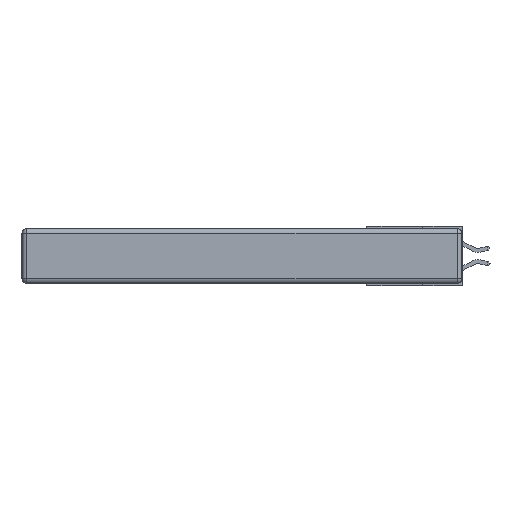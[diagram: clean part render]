
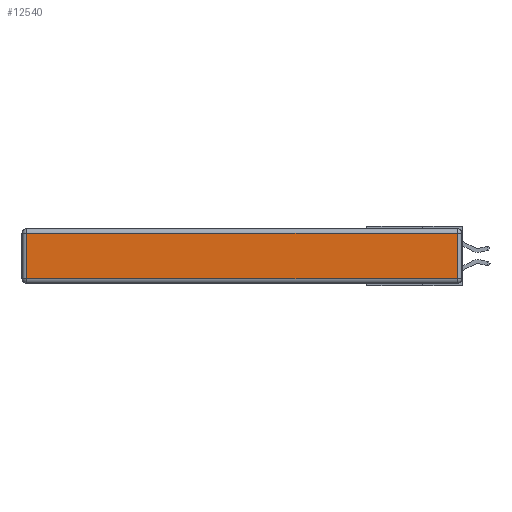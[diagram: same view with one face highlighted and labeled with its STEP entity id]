
A CAD part, left-side view. The second image highlights one B-rep face of the part: STEP entity #12540.
In plain terms, the highlighted planar face has unit normal (-1, 0, 0).
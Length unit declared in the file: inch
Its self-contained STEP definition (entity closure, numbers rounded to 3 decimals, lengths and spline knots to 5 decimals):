
#269 = VERTEX_POINT ( 'NONE', #1005 ) ;
#423 = LINE ( 'NONE', #10934, #9211 ) ;
#887 = LINE ( 'NONE', #6575, #20888 ) ;
#1005 = CARTESIAN_POINT ( 'NONE',  ( 0., 2.72, -0.313 ) ) ;
#1381 = PLANE ( 'NONE',  #4305 ) ;
#2069 = VERTEX_POINT ( 'NONE', #9112 ) ;
#3208 = DIRECTION ( 'NONE',  ( 0., 1., 0. ) ) ;
#3489 = LINE ( 'NONE', #20905, #6738 ) ;
#3576 = EDGE_CURVE ( 'NONE', #2069, #4377, #5082, .T. ) ;
#4305 = AXIS2_PLACEMENT_3D ( 'NONE', #17022, #6510, #20611 ) ;
#4377 = VERTEX_POINT ( 'NONE', #6035 ) ;
#5082 = LINE ( 'NONE', #9165, #8907 ) ;
#6035 = CARTESIAN_POINT ( 'NONE',  ( 0., 0.03, -0.03 ) ) ;
#6452 = ORIENTED_EDGE ( 'NONE', *, *, #16647, .T. ) ;
#6510 = DIRECTION ( 'NONE',  ( -1., 0., 0. ) ) ;
#6575 = CARTESIAN_POINT ( 'NONE',  ( 0., 2.75, -0.03 ) ) ;
#6738 = VECTOR ( 'NONE', #10258, 39.37008 ) ;
#8907 = VECTOR ( 'NONE', #21412, 39.37008 ) ;
#9112 = CARTESIAN_POINT ( 'NONE',  ( 0., 0.03, -0.313 ) ) ;
#9165 = CARTESIAN_POINT ( 'NONE',  ( 0., 0.03, -0.343 ) ) ;
#9211 = VECTOR ( 'NONE', #17987, 39.37008 ) ;
#10258 = DIRECTION ( 'NONE',  ( 0., -1., 0. ) ) ;
#10635 = FACE_OUTER_BOUND ( 'NONE', #21241, .T. ) ;
#10934 = CARTESIAN_POINT ( 'NONE',  ( 0., 2.72, -0.343 ) ) ;
#12540 = ADVANCED_FACE ( 'NONE', ( #10635 ), #1381, .T. ) ;
#13297 = EDGE_CURVE ( 'NONE', #269, #2069, #3489, .T. ) ;
#14236 = ORIENTED_EDGE ( 'NONE', *, *, #19097, .T. ) ;
#14271 = CARTESIAN_POINT ( 'NONE',  ( 0., 2.72, -0.03 ) ) ;
#15314 = ORIENTED_EDGE ( 'NONE', *, *, #13297, .T. ) ;
#15323 = VERTEX_POINT ( 'NONE', #14271 ) ;
#16647 = EDGE_CURVE ( 'NONE', #15323, #269, #423, .T. ) ;
#17022 = CARTESIAN_POINT ( 'NONE',  ( 0., 0., -0.343 ) ) ;
#17987 = DIRECTION ( 'NONE',  ( 0., 0., -1. ) ) ;
#19097 = EDGE_CURVE ( 'NONE', #4377, #15323, #887, .T. ) ;
#19602 = ORIENTED_EDGE ( 'NONE', *, *, #3576, .T. ) ;
#20611 = DIRECTION ( 'NONE',  ( 0., 0., 1. ) ) ;
#20888 = VECTOR ( 'NONE', #3208, 39.37008 ) ;
#20905 = CARTESIAN_POINT ( 'NONE',  ( 0., 0., -0.313 ) ) ;
#21241 = EDGE_LOOP ( 'NONE', ( #15314, #19602, #14236, #6452 ) ) ;
#21412 = DIRECTION ( 'NONE',  ( 0., 0., 1. ) ) ;
